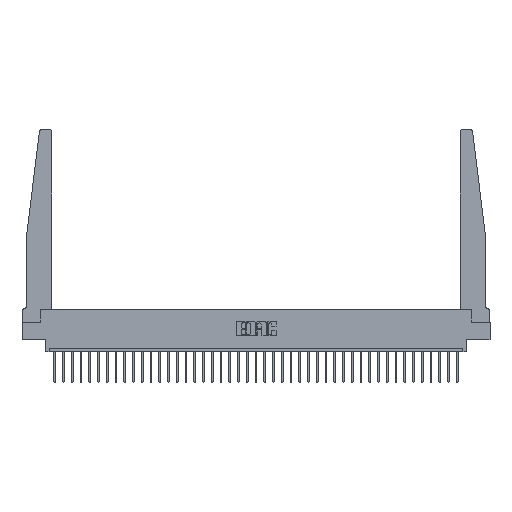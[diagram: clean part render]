
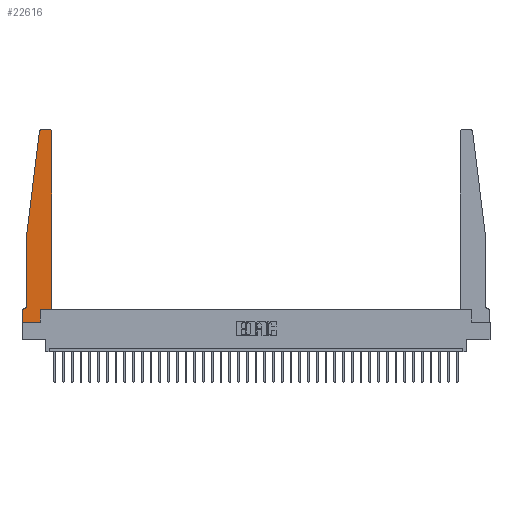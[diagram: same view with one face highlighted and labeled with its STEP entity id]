
A CAD part, top view. The second image highlights one B-rep face of the part: STEP entity #22616.
In plain terms, the highlighted planar face has unit normal (0, 0, 1).
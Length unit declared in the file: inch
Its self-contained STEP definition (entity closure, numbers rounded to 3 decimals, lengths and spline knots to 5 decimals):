
#189 = EDGE_CURVE ( 'NONE', #4295, #26453, #21243, .T. ) ;
#297 = CARTESIAN_POINT ( 'NONE',  ( 0.425, 0.18, 0.37 ) ) ;
#563 = AXIS2_PLACEMENT_3D ( 'NONE', #25732, #9609, #22830 ) ;
#849 = ORIENTED_EDGE ( 'NONE', *, *, #1760, .T. ) ;
#858 = CARTESIAN_POINT ( 'NONE',  ( 0.25, 2.75, 0.37 ) ) ;
#918 = ORIENTED_EDGE ( 'NONE', *, *, #189, .T. ) ;
#1357 = ORIENTED_EDGE ( 'NONE', *, *, #4798, .T. ) ;
#1760 = EDGE_CURVE ( 'NONE', #20806, #29906, #26191, .T. ) ;
#2295 = VERTEX_POINT ( 'NONE', #7791 ) ;
#2607 = AXIS2_PLACEMENT_3D ( 'NONE', #25862, #31311, #20728 ) ;
#3584 = DIRECTION ( 'NONE',  ( 0., 1., 0. ) ) ;
#3988 = ORIENTED_EDGE ( 'NONE', *, *, #31002, .T. ) ;
#4295 = VERTEX_POINT ( 'NONE', #17649 ) ;
#4755 = EDGE_CURVE ( 'NONE', #16525, #15135, #10240, .T. ) ;
#4762 = CARTESIAN_POINT ( 'NONE',  ( 0.395, 2.72, 0.37 ) ) ;
#4798 = EDGE_CURVE ( 'NONE', #29906, #15197, #28035, .T. ) ;
#4933 = DIRECTION ( 'NONE',  ( 1., 0., 0. ) ) ;
#4939 = CARTESIAN_POINT ( 'NONE',  ( 0.2605, 0., 0.37 ) ) ;
#5426 = EDGE_CURVE ( 'NONE', #2295, #16525, #10990, .T. ) ;
#5472 = CARTESIAN_POINT ( 'NONE',  ( 0., 0., 0.37 ) ) ;
#6032 = DIRECTION ( 'NONE',  ( -0.122, -0.992, 0. ) ) ;
#6671 = ORIENTED_EDGE ( 'NONE', *, *, #21408, .T. ) ;
#6852 = ORIENTED_EDGE ( 'NONE', *, *, #18439, .T. ) ;
#6935 = CARTESIAN_POINT ( 'NONE',  ( 0.2605, 0.18, 0.37 ) ) ;
#7003 = DIRECTION ( 'NONE',  ( 0., 0., 1. ) ) ;
#7240 = AXIS2_PLACEMENT_3D ( 'NONE', #4762, #7003, #4933 ) ;
#7576 = ORIENTED_EDGE ( 'NONE', *, *, #4755, .T. ) ;
#7714 = DIRECTION ( 'NONE',  ( 1., 0., 0. ) ) ;
#7791 = CARTESIAN_POINT ( 'NONE',  ( 0.24675, 2.72367, 0.37 ) ) ;
#9246 = ORIENTED_EDGE ( 'NONE', *, *, #5426, .T. ) ;
#9609 = DIRECTION ( 'NONE',  ( 0., 0., 1. ) ) ;
#9758 = DIRECTION ( 'NONE',  ( 1., 0., 0. ) ) ;
#10240 = LINE ( 'NONE', #12814, #19283 ) ;
#10763 = CARTESIAN_POINT ( 'NONE',  ( 0.065, 0.1875, 0.37 ) ) ;
#10990 = LINE ( 'NONE', #11172, #18217 ) ;
#11172 = CARTESIAN_POINT ( 'NONE',  ( 0.065, 1.25, 0.37 ) ) ;
#11374 = EDGE_CURVE ( 'NONE', #15364, #28118, #16600, .T. ) ;
#11574 = ORIENTED_EDGE ( 'NONE', *, *, #26344, .T. ) ;
#12345 = PLANE ( 'NONE',  #563 ) ;
#12814 = CARTESIAN_POINT ( 'NONE',  ( 0.065, 1.25, 0.37 ) ) ;
#12864 = FACE_OUTER_BOUND ( 'NONE', #28252, .T. ) ;
#12935 = VECTOR ( 'NONE', #25901, 39.37008 ) ;
#14774 = VECTOR ( 'NONE', #15727, 39.37008 ) ;
#15135 = VERTEX_POINT ( 'NONE', #15293 ) ;
#15197 = VERTEX_POINT ( 'NONE', #30377 ) ;
#15259 = LINE ( 'NONE', #25731, #12935 ) ;
#15293 = CARTESIAN_POINT ( 'NONE',  ( 0.065, 0.2375, 0.37 ) ) ;
#15364 = VERTEX_POINT ( 'NONE', #23550 ) ;
#15416 = VECTOR ( 'NONE', #31815, 39.37008 ) ;
#15727 = DIRECTION ( 'NONE',  ( 0., 1., 0. ) ) ;
#16525 = VERTEX_POINT ( 'NONE', #28495 ) ;
#16600 = LINE ( 'NONE', #5472, #31530 ) ;
#16976 = EDGE_CURVE ( 'NONE', #26453, #15364, #15259, .T. ) ;
#17304 = CARTESIAN_POINT ( 'NONE',  ( 0.27653, 2.72, 0.37 ) ) ;
#17379 = CIRCLE ( 'NONE', #2607, 0.05 ) ;
#17649 = CARTESIAN_POINT ( 'NONE',  ( 0.015, 0.1875, 0.37 ) ) ;
#18217 = VECTOR ( 'NONE', #6032, 39.37008 ) ;
#18329 = CARTESIAN_POINT ( 'NONE',  ( 0.425, 0.18, 0.37 ) ) ;
#18439 = EDGE_CURVE ( 'NONE', #15135, #4295, #17379, .T. ) ;
#19103 = AXIS2_PLACEMENT_3D ( 'NONE', #17304, #28269, #9758 ) ;
#19283 = VECTOR ( 'NONE', #20717, 39.37008 ) ;
#19365 = CARTESIAN_POINT ( 'NONE',  ( 0.2605, 0.18, 0.37 ) ) ;
#19883 = LINE ( 'NONE', #858, #30828 ) ;
#20401 = VECTOR ( 'NONE', #3584, 39.37008 ) ;
#20717 = DIRECTION ( 'NONE',  ( 0., -1., 0. ) ) ;
#20728 = DIRECTION ( 'NONE',  ( -1., 0., 0. ) ) ;
#20806 = VERTEX_POINT ( 'NONE', #24905 ) ;
#21243 = LINE ( 'NONE', #10763, #15416 ) ;
#21408 = EDGE_CURVE ( 'NONE', #24626, #2295, #31675, .T. ) ;
#21780 = LINE ( 'NONE', #19365, #20401 ) ;
#22127 = DIRECTION ( 'NONE',  ( -1., 0., 0. ) ) ;
#22616 = ADVANCED_FACE ( 'NONE', ( #12864 ), #12345, .T. ) ;
#22830 = DIRECTION ( 'NONE',  ( 1., 0., 0. ) ) ;
#23550 = CARTESIAN_POINT ( 'NONE',  ( 0., 0., 0.37 ) ) ;
#23893 = ORIENTED_EDGE ( 'NONE', *, *, #25668, .T. ) ;
#24168 = CARTESIAN_POINT ( 'NONE',  ( 0., 0.1875, 0.37 ) ) ;
#24626 = VERTEX_POINT ( 'NONE', #29440 ) ;
#24905 = CARTESIAN_POINT ( 'NONE',  ( 0.425, 0.18, 0.37 ) ) ;
#25351 = ORIENTED_EDGE ( 'NONE', *, *, #16976, .T. ) ;
#25668 = EDGE_CURVE ( 'NONE', #28118, #32021, #21780, .T. ) ;
#25723 = LINE ( 'NONE', #18329, #25851 ) ;
#25731 = CARTESIAN_POINT ( 'NONE',  ( 0., 0., 0.37 ) ) ;
#25732 = CARTESIAN_POINT ( 'NONE',  ( 0., 0.1875, 0.37 ) ) ;
#25851 = VECTOR ( 'NONE', #7714, 39.37008 ) ;
#25862 = CARTESIAN_POINT ( 'NONE',  ( 0.015, 0.2375, 0.37 ) ) ;
#25901 = DIRECTION ( 'NONE',  ( 0., -1., 0. ) ) ;
#26191 = LINE ( 'NONE', #297, #14774 ) ;
#26344 = EDGE_CURVE ( 'NONE', #32021, #20806, #25723, .T. ) ;
#26453 = VERTEX_POINT ( 'NONE', #24168 ) ;
#26914 = CARTESIAN_POINT ( 'NONE',  ( 0.425, 2.72, 0.37 ) ) ;
#28035 = CIRCLE ( 'NONE', #7240, 0.03 ) ;
#28118 = VERTEX_POINT ( 'NONE', #4939 ) ;
#28252 = EDGE_LOOP ( 'NONE', ( #3988, #6671, #9246, #7576, #6852, #918, #25351, #31564, #23893, #11574, #849, #1357 ) ) ;
#28269 = DIRECTION ( 'NONE',  ( 0., 0., 1. ) ) ;
#28495 = CARTESIAN_POINT ( 'NONE',  ( 0.065, 1.25, 0.37 ) ) ;
#29440 = CARTESIAN_POINT ( 'NONE',  ( 0.27653, 2.75, 0.37 ) ) ;
#29452 = DIRECTION ( 'NONE',  ( 1., 0., 0. ) ) ;
#29906 = VERTEX_POINT ( 'NONE', #26914 ) ;
#30377 = CARTESIAN_POINT ( 'NONE',  ( 0.395, 2.75, 0.37 ) ) ;
#30828 = VECTOR ( 'NONE', #22127, 39.37008 ) ;
#31002 = EDGE_CURVE ( 'NONE', #15197, #24626, #19883, .T. ) ;
#31311 = DIRECTION ( 'NONE',  ( 0., 0., -1. ) ) ;
#31530 = VECTOR ( 'NONE', #29452, 39.37008 ) ;
#31564 = ORIENTED_EDGE ( 'NONE', *, *, #11374, .T. ) ;
#31675 = CIRCLE ( 'NONE', #19103, 0.03 ) ;
#31815 = DIRECTION ( 'NONE',  ( -1., 0., 0. ) ) ;
#32021 = VERTEX_POINT ( 'NONE', #6935 ) ;
